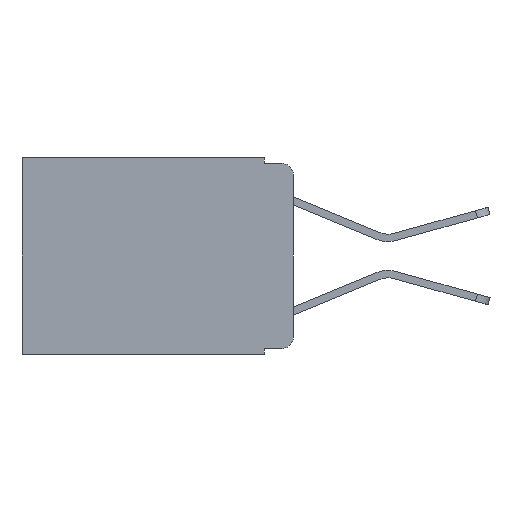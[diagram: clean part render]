
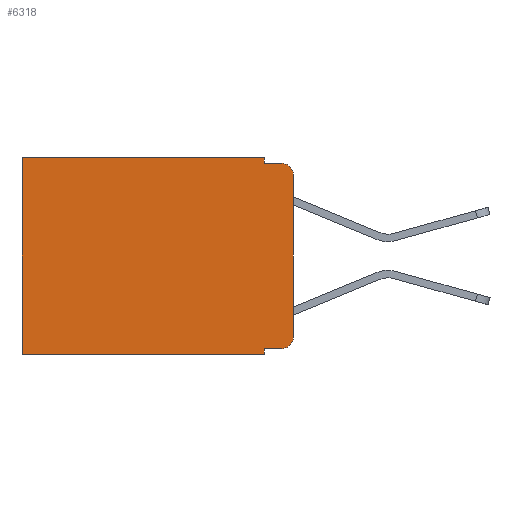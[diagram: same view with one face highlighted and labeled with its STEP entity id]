
A CAD part, left-side view. The second image highlights one B-rep face of the part: STEP entity #6318.
In plain terms, the highlighted planar face has unit normal (-1, 0, 0).
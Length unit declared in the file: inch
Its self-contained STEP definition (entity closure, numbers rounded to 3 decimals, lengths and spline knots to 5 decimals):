
#172 = VECTOR ( 'NONE', #1282, 39.37008 ) ;
#448 = CARTESIAN_POINT ( 'NONE',  ( 0.298, 0.02, -0.313 ) ) ;
#549 = CARTESIAN_POINT ( 'NONE',  ( 0.298, 0., 0. ) ) ;
#627 = CARTESIAN_POINT ( 'NONE',  ( 0.298, 0.02, -0.03 ) ) ;
#728 = VECTOR ( 'NONE', #8494, 39.37008 ) ;
#850 = VECTOR ( 'NONE', #10761, 39.37008 ) ;
#1001 = EDGE_CURVE ( 'NONE', #7068, #2866, #1430, .T. ) ;
#1006 = CARTESIAN_POINT ( 'NONE',  ( 0.298, 0., 0. ) ) ;
#1027 = ORIENTED_EDGE ( 'NONE', *, *, #1617, .F. ) ;
#1282 = DIRECTION ( 'NONE',  ( 0., 0., -1. ) ) ;
#1360 = DIRECTION ( 'NONE',  ( 0., 0., -1. ) ) ;
#1396 = CARTESIAN_POINT ( 'NONE',  ( 0.298, 0., -0.03 ) ) ;
#1430 = LINE ( 'NONE', #2381, #5441 ) ;
#1554 = CARTESIAN_POINT ( 'NONE',  ( 0.298, 0.051, -0.01 ) ) ;
#1617 = EDGE_CURVE ( 'NONE', #4182, #8838, #1974, .T. ) ;
#1974 = LINE ( 'NONE', #7914, #9462 ) ;
#2093 = VERTEX_POINT ( 'NONE', #9845 ) ;
#2118 = CARTESIAN_POINT ( 'NONE',  ( 0.298, 0.473, -0.343 ) ) ;
#2216 = EDGE_CURVE ( 'NONE', #7610, #8838, #9900, .T. ) ;
#2297 = DIRECTION ( 'NONE',  ( 0., 0., -1. ) ) ;
#2381 = CARTESIAN_POINT ( 'NONE',  ( 0.298, 0.051, -0.333 ) ) ;
#2465 = AXIS2_PLACEMENT_3D ( 'NONE', #627, #9735, #7109 ) ;
#2661 = DIRECTION ( 'NONE',  ( 0., 0., -1. ) ) ;
#2866 = VERTEX_POINT ( 'NONE', #10274 ) ;
#2965 = CARTESIAN_POINT ( 'NONE',  ( 0.298, 0.051, 0. ) ) ;
#3400 = ORIENTED_EDGE ( 'NONE', *, *, #9360, .F. ) ;
#3483 = ORIENTED_EDGE ( 'NONE', *, *, #5228, .T. ) ;
#3679 = VECTOR ( 'NONE', #7400, 39.37008 ) ;
#3810 = EDGE_CURVE ( 'NONE', #8823, #2093, #6256, .T. ) ;
#3863 = EDGE_LOOP ( 'NONE', ( #8688, #4259, #8601, #9046, #3483, #7439, #1027, #3400, #6522, #10078 ) ) ;
#4182 = VERTEX_POINT ( 'NONE', #7049 ) ;
#4222 = PLANE ( 'NONE',  #4555 ) ;
#4259 = ORIENTED_EDGE ( 'NONE', *, *, #3810, .T. ) ;
#4294 = LINE ( 'NONE', #8850, #850 ) ;
#4353 = LINE ( 'NONE', #8647, #172 ) ;
#4555 = AXIS2_PLACEMENT_3D ( 'NONE', #549, #8791, #1360 ) ;
#4696 = VECTOR ( 'NONE', #9295, 39.37008 ) ;
#5228 = EDGE_CURVE ( 'NONE', #11854, #7610, #11135, .T. ) ;
#5250 = CARTESIAN_POINT ( 'NONE',  ( 0.298, 0.051, -0.333 ) ) ;
#5441 = VECTOR ( 'NONE', #10595, 39.37008 ) ;
#5600 = CIRCLE ( 'NONE', #11811, 0.02 ) ;
#5946 = CARTESIAN_POINT ( 'NONE',  ( 0.298, 0.473, 0. ) ) ;
#6243 = CARTESIAN_POINT ( 'NONE',  ( 0.298, 0.473, 0. ) ) ;
#6256 = CIRCLE ( 'NONE', #2465, 0.02 ) ;
#6318 = ADVANCED_FACE ( 'NONE', ( #9334 ), #4222, .F. ) ;
#6522 = ORIENTED_EDGE ( 'NONE', *, *, #1001, .T. ) ;
#7023 = DIRECTION ( 'NONE',  ( -1., 0., 0. ) ) ;
#7049 = CARTESIAN_POINT ( 'NONE',  ( 0.298, 0.051, -0.343 ) ) ;
#7068 = VERTEX_POINT ( 'NONE', #5250 ) ;
#7109 = DIRECTION ( 'NONE',  ( 0., 0., -1. ) ) ;
#7338 = EDGE_CURVE ( 'NONE', #8823, #10932, #4353, .T. ) ;
#7400 = DIRECTION ( 'NONE',  ( 0., 1., 0. ) ) ;
#7439 = ORIENTED_EDGE ( 'NONE', *, *, #2216, .T. ) ;
#7459 = LINE ( 'NONE', #11079, #9772 ) ;
#7610 = VERTEX_POINT ( 'NONE', #6243 ) ;
#7914 = CARTESIAN_POINT ( 'NONE',  ( 0.298, 0., -0.343 ) ) ;
#8374 = EDGE_CURVE ( 'NONE', #2866, #10932, #5600, .T. ) ;
#8492 = EDGE_CURVE ( 'NONE', #11854, #9583, #7459, .T. ) ;
#8494 = DIRECTION ( 'NONE',  ( 0., 0., -1. ) ) ;
#8601 = ORIENTED_EDGE ( 'NONE', *, *, #10237, .F. ) ;
#8647 = CARTESIAN_POINT ( 'NONE',  ( 0.298, 0., 0. ) ) ;
#8688 = ORIENTED_EDGE ( 'NONE', *, *, #7338, .F. ) ;
#8791 = DIRECTION ( 'NONE',  ( 1., 0., 0. ) ) ;
#8823 = VERTEX_POINT ( 'NONE', #1396 ) ;
#8838 = VERTEX_POINT ( 'NONE', #2118 ) ;
#8850 = CARTESIAN_POINT ( 'NONE',  ( 0.298, 0.051, -0.01 ) ) ;
#9046 = ORIENTED_EDGE ( 'NONE', *, *, #8492, .F. ) ;
#9292 = CARTESIAN_POINT ( 'NONE',  ( 0.298, 0.051, 0. ) ) ;
#9295 = DIRECTION ( 'NONE',  ( 0., 0., -1. ) ) ;
#9334 = FACE_OUTER_BOUND ( 'NONE', #3863, .T. ) ;
#9343 = LINE ( 'NONE', #2965, #728 ) ;
#9360 = EDGE_CURVE ( 'NONE', #7068, #4182, #9343, .T. ) ;
#9462 = VECTOR ( 'NONE', #9630, 39.37008 ) ;
#9583 = VERTEX_POINT ( 'NONE', #1554 ) ;
#9630 = DIRECTION ( 'NONE',  ( 0., 1., 0. ) ) ;
#9735 = DIRECTION ( 'NONE',  ( -1., 0., 0. ) ) ;
#9772 = VECTOR ( 'NONE', #2661, 39.37008 ) ;
#9845 = CARTESIAN_POINT ( 'NONE',  ( 0.298, 0.02, -0.01 ) ) ;
#9900 = LINE ( 'NONE', #5946, #4696 ) ;
#10078 = ORIENTED_EDGE ( 'NONE', *, *, #8374, .T. ) ;
#10237 = EDGE_CURVE ( 'NONE', #9583, #2093, #4294, .T. ) ;
#10274 = CARTESIAN_POINT ( 'NONE',  ( 0.298, 0.02, -0.333 ) ) ;
#10595 = DIRECTION ( 'NONE',  ( 0., -1., 0. ) ) ;
#10748 = CARTESIAN_POINT ( 'NONE',  ( 0.298, 0., -0.313 ) ) ;
#10761 = DIRECTION ( 'NONE',  ( 0., -1., 0. ) ) ;
#10932 = VERTEX_POINT ( 'NONE', #10748 ) ;
#11079 = CARTESIAN_POINT ( 'NONE',  ( 0.298, 0.051, 0. ) ) ;
#11135 = LINE ( 'NONE', #1006, #3679 ) ;
#11811 = AXIS2_PLACEMENT_3D ( 'NONE', #448, #7023, #2297 ) ;
#11854 = VERTEX_POINT ( 'NONE', #9292 ) ;
